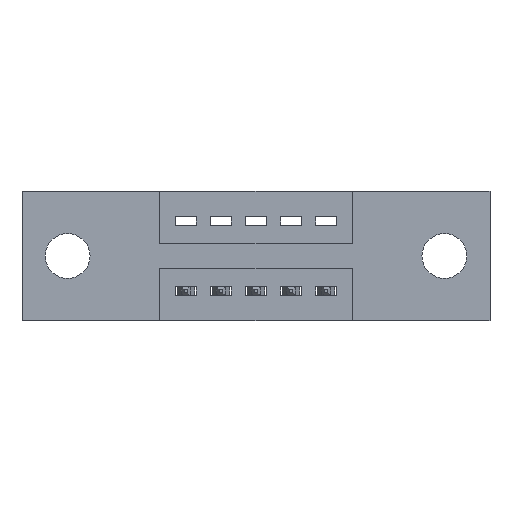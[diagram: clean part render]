
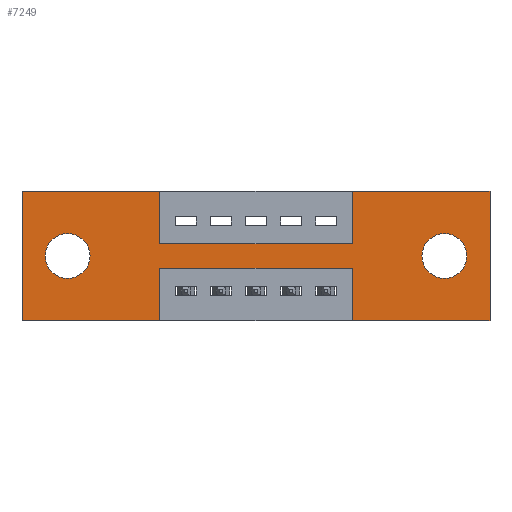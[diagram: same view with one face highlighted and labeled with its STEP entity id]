
A CAD part, front view. The second image highlights one B-rep face of the part: STEP entity #7249.
In plain terms, the highlighted planar face has unit normal (0, -1, 0).
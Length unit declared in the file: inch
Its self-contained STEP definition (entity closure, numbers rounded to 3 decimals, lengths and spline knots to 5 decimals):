
#17 = CIRCLE ( 'NONE', #4799, 0.064 ) ;
#35 = CIRCLE ( 'NONE', #2056, 0.064 ) ;
#87 = VERTEX_POINT ( 'NONE', #3997 ) ;
#144 = CARTESIAN_POINT ( 'NONE',  ( 0., 0., 0. ) ) ;
#186 = CARTESIAN_POINT ( 'NONE',  ( 1.205, 0., -0.185 ) ) ;
#206 = CARTESIAN_POINT ( 'NONE',  ( 1.335, 0., 0. ) ) ;
#351 = VERTEX_POINT ( 'NONE', #7701 ) ;
#619 = DIRECTION ( 'NONE',  ( 0., 1., 0. ) ) ;
#758 = VECTOR ( 'NONE', #2643, 39.37008 ) ;
#764 = LINE ( 'NONE', #144, #2379 ) ;
#805 = CARTESIAN_POINT ( 'NONE',  ( 0.13, 0., -0.185 ) ) ;
#867 = EDGE_CURVE ( 'NONE', #87, #5846, #6151, .T. ) ;
#891 = DIRECTION ( 'NONE',  ( 0., 0., -1. ) ) ;
#1019 = ORIENTED_EDGE ( 'NONE', *, *, #3149, .F. ) ;
#1022 = EDGE_CURVE ( 'NONE', #3625, #6349, #7796, .T. ) ;
#1137 = CARTESIAN_POINT ( 'NONE',  ( 0.9425, 0., -0.37 ) ) ;
#1243 = VERTEX_POINT ( 'NONE', #1419 ) ;
#1255 = EDGE_LOOP ( 'NONE', ( #5909, #6531 ) ) ;
#1269 = EDGE_LOOP ( 'NONE', ( #1019, #1464, #7252, #7671, #2952, #6023, #8221, #6659, #5723, #2233, #7371, #1486 ) ) ;
#1334 = EDGE_CURVE ( 'NONE', #8632, #1243, #8649, .T. ) ;
#1419 = CARTESIAN_POINT ( 'NONE',  ( 0.13, 0., -0.121 ) ) ;
#1460 = CARTESIAN_POINT ( 'NONE',  ( 0., 0., 0. ) ) ;
#1464 = ORIENTED_EDGE ( 'NONE', *, *, #2516, .F. ) ;
#1474 = CARTESIAN_POINT ( 'NONE',  ( 1.205, 0., -0.121 ) ) ;
#1486 = ORIENTED_EDGE ( 'NONE', *, *, #3077, .F. ) ;
#1500 = DIRECTION ( 'NONE',  ( 0., 0., 1. ) ) ;
#1521 = AXIS2_PLACEMENT_3D ( 'NONE', #8192, #8042, #8032 ) ;
#1524 = LINE ( 'NONE', #1460, #3105 ) ;
#1721 = CARTESIAN_POINT ( 'NONE',  ( 0.3925, 0., 0. ) ) ;
#1751 = EDGE_CURVE ( 'NONE', #6349, #4545, #6322, .T. ) ;
#2014 = CARTESIAN_POINT ( 'NONE',  ( 0., 0., 0. ) ) ;
#2056 = AXIS2_PLACEMENT_3D ( 'NONE', #186, #4968, #891 ) ;
#2221 = ORIENTED_EDGE ( 'NONE', *, *, #1334, .T. ) ;
#2233 = ORIENTED_EDGE ( 'NONE', *, *, #8105, .F. ) ;
#2359 = VERTEX_POINT ( 'NONE', #5641 ) ;
#2373 = DIRECTION ( 'NONE',  ( 1., 0., 0. ) ) ;
#2379 = VECTOR ( 'NONE', #6264, 39.37008 ) ;
#2425 = VERTEX_POINT ( 'NONE', #4366 ) ;
#2486 = LINE ( 'NONE', #3708, #3866 ) ;
#2516 = EDGE_CURVE ( 'NONE', #5846, #5224, #8714, .T. ) ;
#2572 = FACE_BOUND ( 'NONE', #1255, .T. ) ;
#2600 = CARTESIAN_POINT ( 'NONE',  ( 0., 0., -0.37 ) ) ;
#2643 = DIRECTION ( 'NONE',  ( 0., 0., 1. ) ) ;
#2875 = VERTEX_POINT ( 'NONE', #1474 ) ;
#2952 = ORIENTED_EDGE ( 'NONE', *, *, #4284, .F. ) ;
#3030 = CARTESIAN_POINT ( 'NONE',  ( 0.9425, 0., 0. ) ) ;
#3067 = CARTESIAN_POINT ( 'NONE',  ( 0.3925, 0., -0.37 ) ) ;
#3077 = EDGE_CURVE ( 'NONE', #2359, #5926, #8081, .T. ) ;
#3105 = VECTOR ( 'NONE', #6201, 39.37008 ) ;
#3149 = EDGE_CURVE ( 'NONE', #5224, #2359, #5898, .T. ) ;
#3204 = CARTESIAN_POINT ( 'NONE',  ( 0.3925, 0., -0.22 ) ) ;
#3476 = DIRECTION ( 'NONE',  ( 1., 0., 0. ) ) ;
#3551 = LINE ( 'NONE', #206, #6917 ) ;
#3559 = CARTESIAN_POINT ( 'NONE',  ( 0.3925, 0., -0.15 ) ) ;
#3625 = VERTEX_POINT ( 'NONE', #4261 ) ;
#3638 = EDGE_CURVE ( 'NONE', #351, #2875, #35, .T. ) ;
#3671 = AXIS2_PLACEMENT_3D ( 'NONE', #805, #5570, #1500 ) ;
#3708 = CARTESIAN_POINT ( 'NONE',  ( 0., 0., 0. ) ) ;
#3866 = VECTOR ( 'NONE', #2373, 39.37008 ) ;
#3916 = VERTEX_POINT ( 'NONE', #5924 ) ;
#3965 = LINE ( 'NONE', #2600, #7314 ) ;
#3997 = CARTESIAN_POINT ( 'NONE',  ( 0.9425, 0., -0.37 ) ) ;
#4007 = DIRECTION ( 'NONE',  ( 0., -1., 0. ) ) ;
#4074 = CIRCLE ( 'NONE', #3671, 0.064 ) ;
#4261 = CARTESIAN_POINT ( 'NONE',  ( 0.3925, 0., 0. ) ) ;
#4284 = EDGE_CURVE ( 'NONE', #2425, #3916, #3551, .T. ) ;
#4366 = CARTESIAN_POINT ( 'NONE',  ( 1.335, 0., 0. ) ) ;
#4384 = CARTESIAN_POINT ( 'NONE',  ( 0., 0., -0.37 ) ) ;
#4386 = FACE_BOUND ( 'NONE', #5929, .T. ) ;
#4532 = VECTOR ( 'NONE', #5067, 39.37008 ) ;
#4534 = VECTOR ( 'NONE', #3476, 39.37008 ) ;
#4545 = VERTEX_POINT ( 'NONE', #5261 ) ;
#4621 = DIRECTION ( 'NONE',  ( -1., 0., 0. ) ) ;
#4704 = CARTESIAN_POINT ( 'NONE',  ( 0.9425, 0., 0. ) ) ;
#4719 = CARTESIAN_POINT ( 'NONE',  ( 1.205, 0., -0.185 ) ) ;
#4799 = AXIS2_PLACEMENT_3D ( 'NONE', #4719, #619, #5397 ) ;
#4968 = DIRECTION ( 'NONE',  ( 0., 1., 0. ) ) ;
#4986 = DIRECTION ( 'NONE',  ( 0., 0., -1. ) ) ;
#5067 = DIRECTION ( 'NONE',  ( -1., 0., 0. ) ) ;
#5138 = CARTESIAN_POINT ( 'NONE',  ( 0.3925, 0., -0.22 ) ) ;
#5224 = VERTEX_POINT ( 'NONE', #3204 ) ;
#5225 = CARTESIAN_POINT ( 'NONE',  ( 0.9425, 0., -0.22 ) ) ;
#5261 = CARTESIAN_POINT ( 'NONE',  ( 0.9425, 0., -0.15 ) ) ;
#5397 = DIRECTION ( 'NONE',  ( 0., 0., -1. ) ) ;
#5570 = DIRECTION ( 'NONE',  ( 0., 1., 0. ) ) ;
#5641 = CARTESIAN_POINT ( 'NONE',  ( 0.3925, 0., -0.37 ) ) ;
#5693 = VECTOR ( 'NONE', #7102, 39.37008 ) ;
#5723 = ORIENTED_EDGE ( 'NONE', *, *, #1022, .F. ) ;
#5846 = VERTEX_POINT ( 'NONE', #5225 ) ;
#5898 = LINE ( 'NONE', #3067, #5693 ) ;
#5909 = ORIENTED_EDGE ( 'NONE', *, *, #6018, .T. ) ;
#5924 = CARTESIAN_POINT ( 'NONE',  ( 1.335, 0., -0.37 ) ) ;
#5926 = VERTEX_POINT ( 'NONE', #8639 ) ;
#5929 = EDGE_LOOP ( 'NONE', ( #6958, #2221 ) ) ;
#5962 = LINE ( 'NONE', #4704, #758 ) ;
#6014 = PLANE ( 'NONE',  #8089 ) ;
#6018 = EDGE_CURVE ( 'NONE', #2875, #351, #17, .T. ) ;
#6023 = ORIENTED_EDGE ( 'NONE', *, *, #6841, .F. ) ;
#6024 = VERTEX_POINT ( 'NONE', #2014 ) ;
#6151 = LINE ( 'NONE', #1137, #8657 ) ;
#6201 = DIRECTION ( 'NONE',  ( 0., 0., 1. ) ) ;
#6264 = DIRECTION ( 'NONE',  ( 1., 0., 0. ) ) ;
#6322 = LINE ( 'NONE', #3559, #4534 ) ;
#6349 = VERTEX_POINT ( 'NONE', #7738 ) ;
#6531 = ORIENTED_EDGE ( 'NONE', *, *, #3638, .T. ) ;
#6659 = ORIENTED_EDGE ( 'NONE', *, *, #1751, .F. ) ;
#6841 = EDGE_CURVE ( 'NONE', #7548, #2425, #764, .T. ) ;
#6917 = VECTOR ( 'NONE', #4986, 39.37008 ) ;
#6930 = VECTOR ( 'NONE', #7141, 39.37008 ) ;
#6958 = ORIENTED_EDGE ( 'NONE', *, *, #8566, .T. ) ;
#7102 = DIRECTION ( 'NONE',  ( 0., 0., -1. ) ) ;
#7141 = DIRECTION ( 'NONE',  ( -1., 0., 0. ) ) ;
#7249 = ADVANCED_FACE ( 'NONE', ( #2572, #4386, #7936 ), #6014, .T. ) ;
#7252 = ORIENTED_EDGE ( 'NONE', *, *, #867, .F. ) ;
#7254 = EDGE_CURVE ( 'NONE', #4545, #7548, #5962, .T. ) ;
#7314 = VECTOR ( 'NONE', #4621, 39.37008 ) ;
#7371 = ORIENTED_EDGE ( 'NONE', *, *, #7379, .F. ) ;
#7372 = VECTOR ( 'NONE', #7674, 39.37008 ) ;
#7379 = EDGE_CURVE ( 'NONE', #5926, #6024, #1524, .T. ) ;
#7457 = DIRECTION ( 'NONE',  ( 0., 0., 1. ) ) ;
#7548 = VERTEX_POINT ( 'NONE', #3030 ) ;
#7671 = ORIENTED_EDGE ( 'NONE', *, *, #8330, .F. ) ;
#7674 = DIRECTION ( 'NONE',  ( 0., 0., -1. ) ) ;
#7701 = CARTESIAN_POINT ( 'NONE',  ( 1.205, 0., -0.249 ) ) ;
#7738 = CARTESIAN_POINT ( 'NONE',  ( 0.3925, 0., -0.15 ) ) ;
#7796 = LINE ( 'NONE', #1721, #7372 ) ;
#7936 = FACE_OUTER_BOUND ( 'NONE', #1269, .T. ) ;
#8015 = CARTESIAN_POINT ( 'NONE',  ( 0., 0., -0.37 ) ) ;
#8032 = DIRECTION ( 'NONE',  ( 0., 0., 1. ) ) ;
#8042 = DIRECTION ( 'NONE',  ( 0., 1., 0. ) ) ;
#8081 = LINE ( 'NONE', #4384, #4532 ) ;
#8089 = AXIS2_PLACEMENT_3D ( 'NONE', #8015, #4007, #8719 ) ;
#8105 = EDGE_CURVE ( 'NONE', #6024, #3625, #2486, .T. ) ;
#8192 = CARTESIAN_POINT ( 'NONE',  ( 0.13, 0., -0.185 ) ) ;
#8221 = ORIENTED_EDGE ( 'NONE', *, *, #7254, .F. ) ;
#8247 = CARTESIAN_POINT ( 'NONE',  ( 0.13, 0., -0.249 ) ) ;
#8330 = EDGE_CURVE ( 'NONE', #3916, #87, #3965, .T. ) ;
#8566 = EDGE_CURVE ( 'NONE', #1243, #8632, #4074, .T. ) ;
#8632 = VERTEX_POINT ( 'NONE', #8247 ) ;
#8639 = CARTESIAN_POINT ( 'NONE',  ( 0., 0., -0.37 ) ) ;
#8649 = CIRCLE ( 'NONE', #1521, 0.064 ) ;
#8657 = VECTOR ( 'NONE', #7457, 39.37008 ) ;
#8714 = LINE ( 'NONE', #5138, #6930 ) ;
#8719 = DIRECTION ( 'NONE',  ( 0., 0., -1. ) ) ;
